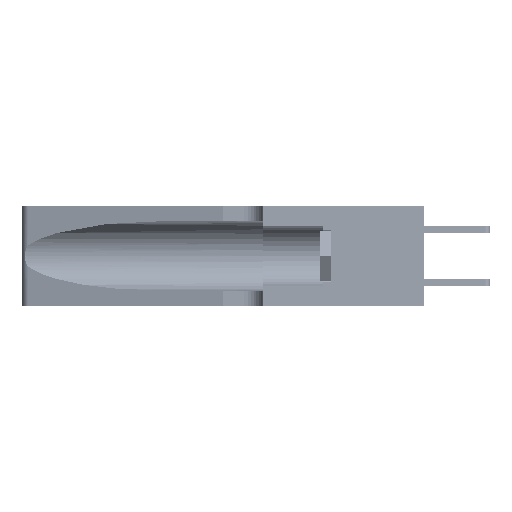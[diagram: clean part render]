
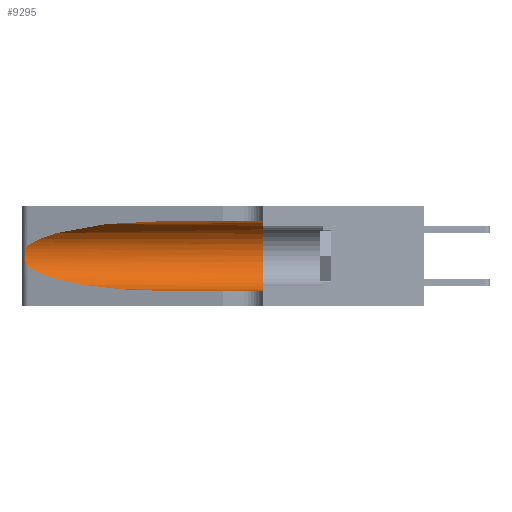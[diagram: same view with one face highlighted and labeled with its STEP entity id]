
A CAD part, left-side view. The second image highlights one B-rep face of the part: STEP entity #9295.
In plain terms, the highlighted cylindrical face has radius 3.308 mm (diameter 6.617 mm), a partial arc.
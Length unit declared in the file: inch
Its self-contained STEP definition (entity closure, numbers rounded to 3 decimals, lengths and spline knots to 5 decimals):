
#47 = EDGE_CURVE ( 'NONE', #10665, #21504, #28135, .T. ) ;
#643 = CARTESIAN_POINT ( 'NONE',  ( 0.25639, 1.23184, 0.21858 ) ) ;
#1187 = CARTESIAN_POINT ( 'NONE',  ( 0.1305, 0.35, 0.05475 ) ) ;
#2990 = CARTESIAN_POINT ( 'NONE',  ( 0.25639, 1.23186, 0.15144 ) ) ;
#3743 = CARTESIAN_POINT ( 'NONE',  ( 0.1305, 0.35, 0.185 ) ) ;
#4447 = DIRECTION ( 'NONE',  ( 0., -1., 0. ) ) ;
#4965 = CARTESIAN_POINT ( 'NONE',  ( 0.25487, 1.22718, 0.14631 ) ) ;
#5705 =( BOUNDED_CURVE ( )  B_SPLINE_CURVE ( 3, ( #28483, #19743, #9948, #28744 ),
 .UNSPECIFIED., .F., .F. ) 
 B_SPLINE_CURVE_WITH_KNOTS ( ( 4, 4 ),
 ( 3.44316, 4.71239 ),
 .UNSPECIFIED. ) 
 CURVE ( )  GEOMETRIC_REPRESENTATION_ITEM ( )  RATIONAL_B_SPLINE_CURVE ( ( 1., 0.87, 0.87, 1. ) ) 
 REPRESENTATION_ITEM ( '' )  );
#7112 = CARTESIAN_POINT ( 'NONE',  ( 0.1305, 0.72297, 0.05475 ) ) ;
#7580 = ORIENTED_EDGE ( 'NONE', *, *, #25036, .F. ) ;
#7945 = FACE_OUTER_BOUND ( 'NONE', #33190, .T. ) ;
#8272 = ORIENTED_EDGE ( 'NONE', *, *, #47, .T. ) ;
#9228 = VECTOR ( 'NONE', #13426, 39.37008 ) ;
#9295 = ADVANCED_FACE ( 'NONE', ( #7945 ), #33007, .F. ) ;
#9601 = CARTESIAN_POINT ( 'NONE',  ( 0.2373, 1.15595, 0.28018 ) ) ;
#9723 = DIRECTION ( 'NONE',  ( 0., 1., 0. ) ) ;
#9948 = CARTESIAN_POINT ( 'NONE',  ( 0.18966, 0.96281, 0.05475 ) ) ;
#10665 = VERTEX_POINT ( 'NONE', #7112 ) ;
#11587 = AXIS2_PLACEMENT_3D ( 'NONE', #35538, #4447, #20827 ) ;
#11660 = ORIENTED_EDGE ( 'NONE', *, *, #18517, .F. ) ;
#11971 = CARTESIAN_POINT ( 'NONE',  ( 0.25555, 1.22993, 0.14849 ) ) ;
#12969 = CIRCLE ( 'NONE', #35685, 0.13025 ) ;
#13190 = VERTEX_POINT ( 'NONE', #4965 ) ;
#13426 = DIRECTION ( 'NONE',  ( 0., -1., 0. ) ) ;
#14163 = B_SPLINE_CURVE_WITH_KNOTS ( 'NONE', 3,
 ( #28774, #26063, #643, #24769, #29731, #26229, #29699, #22419, #17683, #27530, #21760, #2990, #11971, #28063 ),
 .UNSPECIFIED., .F., .F.,
 ( 4, 2, 2, 2, 2, 2, 4 ),
 ( 0., 0.00027, 0.00053, 0.00107, 0.0016, 0.00187, 0.00214 ),
 .UNSPECIFIED. ) ;
#14849 = EDGE_CURVE ( 'NONE', #38607, #35164, #34567, .T. ) ;
#15731 = CARTESIAN_POINT ( 'NONE',  ( 0.25487, 1.22718, 0.22369 ) ) ;
#16292 = ORIENTED_EDGE ( 'NONE', *, *, #16890, .T. ) ;
#16890 = EDGE_CURVE ( 'NONE', #35164, #13190, #14163, .T. ) ;
#17482 = LINE ( 'NONE', #31652, #9228 ) ;
#17683 = CARTESIAN_POINT ( 'NONE',  ( 0.26017, 1.23833, 0.17102 ) ) ;
#18517 = EDGE_CURVE ( 'NONE', #38607, #34807, #17482, .T. ) ;
#19125 = CARTESIAN_POINT ( 'NONE',  ( 0.1305, 1.61858, 0.05475 ) ) ;
#19743 = CARTESIAN_POINT ( 'NONE',  ( 0.2373, 1.15595, 0.08982 ) ) ;
#20348 = ORIENTED_EDGE ( 'NONE', *, *, #24875, .T. ) ;
#20827 = DIRECTION ( 'NONE',  ( 0., 0., -1. ) ) ;
#21504 = VERTEX_POINT ( 'NONE', #1187 ) ;
#21760 = CARTESIAN_POINT ( 'NONE',  ( 0.25789, 1.23486, 0.15765 ) ) ;
#22419 = CARTESIAN_POINT ( 'NONE',  ( 0.26075, 1.23896, 0.178 ) ) ;
#22508 = CARTESIAN_POINT ( 'NONE',  ( 0.1305, 0.72297, 0.31525 ) ) ;
#24769 = CARTESIAN_POINT ( 'NONE',  ( 0.25787, 1.23484, 0.2124 ) ) ;
#24875 = EDGE_CURVE ( 'NONE', #13190, #10665, #5705, .T. ) ;
#25036 = EDGE_CURVE ( 'NONE', #34807, #21504, #12969, .T. ) ;
#25596 = CARTESIAN_POINT ( 'NONE',  ( 0.1305, 0.72297, 0.31525 ) ) ;
#26063 = CARTESIAN_POINT ( 'NONE',  ( 0.25555, 1.22994, 0.2215 ) ) ;
#26229 = CARTESIAN_POINT ( 'NONE',  ( 0.26018, 1.23835, 0.19895 ) ) ;
#27091 = CARTESIAN_POINT ( 'NONE',  ( 0.25487, 1.22718, 0.22369 ) ) ;
#27530 = CARTESIAN_POINT ( 'NONE',  ( 0.25856, 1.23593, 0.16098 ) ) ;
#28063 = CARTESIAN_POINT ( 'NONE',  ( 0.25487, 1.22718, 0.14631 ) ) ;
#28135 = LINE ( 'NONE', #19125, #36318 ) ;
#28455 = ORIENTED_EDGE ( 'NONE', *, *, #14849, .T. ) ;
#28483 = CARTESIAN_POINT ( 'NONE',  ( 0.25487, 1.22718, 0.14631 ) ) ;
#28529 = DIRECTION ( 'NONE',  ( 0., -1., 0. ) ) ;
#28744 = CARTESIAN_POINT ( 'NONE',  ( 0.1305, 0.72297, 0.05475 ) ) ;
#28774 = CARTESIAN_POINT ( 'NONE',  ( 0.25487, 1.22718, 0.22369 ) ) ;
#29699 = CARTESIAN_POINT ( 'NONE',  ( 0.26075, 1.23896, 0.19203 ) ) ;
#29731 = CARTESIAN_POINT ( 'NONE',  ( 0.25854, 1.2359, 0.20912 ) ) ;
#31652 = CARTESIAN_POINT ( 'NONE',  ( 0.1305, 1.61858, 0.31525 ) ) ;
#33007 = CYLINDRICAL_SURFACE ( 'NONE', #11587, 0.13025 ) ;
#33190 = EDGE_LOOP ( 'NONE', ( #28455, #16292, #20348, #8272, #7580, #11660 ) ) ;
#34340 = CARTESIAN_POINT ( 'NONE',  ( 0.18966, 0.96281, 0.31525 ) ) ;
#34567 =( BOUNDED_CURVE ( )  B_SPLINE_CURVE ( 3, ( #22508, #34340, #9601, #15731 ),
 .UNSPECIFIED., .F., .T. ) 
 B_SPLINE_CURVE_WITH_KNOTS ( ( 4, 4 ),
 ( 1.5708, 2.84003 ),
 .UNSPECIFIED. ) 
 CURVE ( )  GEOMETRIC_REPRESENTATION_ITEM ( )  RATIONAL_B_SPLINE_CURVE ( ( 1., 0.87, 0.87, 1. ) ) 
 REPRESENTATION_ITEM ( '' )  );
#34807 = VERTEX_POINT ( 'NONE', #37298 ) ;
#35164 = VERTEX_POINT ( 'NONE', #27091 ) ;
#35538 = CARTESIAN_POINT ( 'NONE',  ( 0.1305, 1.61858, 0.185 ) ) ;
#35685 = AXIS2_PLACEMENT_3D ( 'NONE', #3743, #9723, #37800 ) ;
#36318 = VECTOR ( 'NONE', #28529, 39.37008 ) ;
#37298 = CARTESIAN_POINT ( 'NONE',  ( 0.1305, 0.35, 0.31525 ) ) ;
#37800 = DIRECTION ( 'NONE',  ( 0., 0., 1. ) ) ;
#38607 = VERTEX_POINT ( 'NONE', #25596 ) ;
